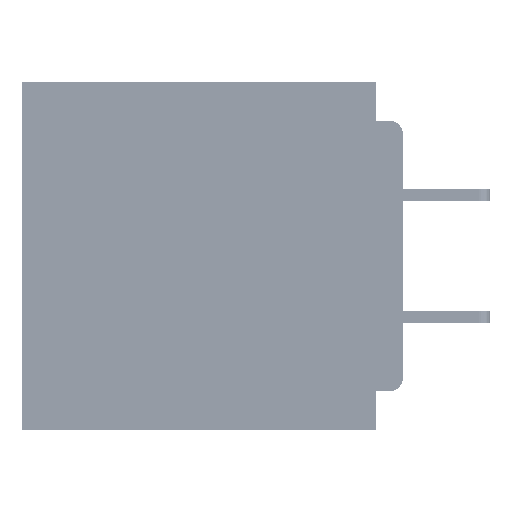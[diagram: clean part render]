
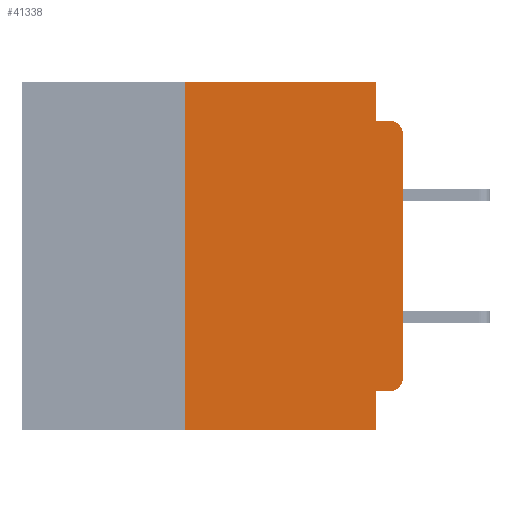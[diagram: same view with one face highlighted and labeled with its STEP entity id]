
A CAD part, left-side view. The second image highlights one B-rep face of the part: STEP entity #41338.
In plain terms, the highlighted planar face has unit normal (-1, 0, 0).
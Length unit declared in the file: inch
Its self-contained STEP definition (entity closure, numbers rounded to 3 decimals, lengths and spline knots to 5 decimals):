
#2596 = LINE ( 'NONE', #50069, #58833 ) ;
#3687 = DIRECTION ( 'NONE',  ( 0., 0., -1. ) ) ;
#3823 = CIRCLE ( 'NONE', #4908, 0.015 ) ;
#4255 = VERTEX_POINT ( 'NONE', #46922 ) ;
#4647 = DIRECTION ( 'NONE',  ( 0., 0., 1. ) ) ;
#4908 = AXIS2_PLACEMENT_3D ( 'NONE', #70573, #38184, #5376 ) ;
#5376 = DIRECTION ( 'NONE',  ( 0., 0., -1. ) ) ;
#5765 = VECTOR ( 'NONE', #49019, 39.37008 ) ;
#6104 = VECTOR ( 'NONE', #42588, 39.37008 ) ;
#8023 = VERTEX_POINT ( 'NONE', #57097 ) ;
#11063 = ORIENTED_EDGE ( 'NONE', *, *, #49867, .T. ) ;
#13191 = ORIENTED_EDGE ( 'NONE', *, *, #67345, .F. ) ;
#15034 = CIRCLE ( 'NONE', #28139, 0.015 ) ;
#16459 = CARTESIAN_POINT ( 'NONE',  ( 0., 0.25, -0.4 ) ) ;
#16585 = EDGE_LOOP ( 'NONE', ( #11063, #57683, #36805, #46174, #51348, #13191, #30051, #34677, #66850, #38359 ) ) ;
#17734 = DIRECTION ( 'NONE',  ( 1., 0., 0. ) ) ;
#17931 = VECTOR ( 'NONE', #3687, 39.37008 ) ;
#18773 = CARTESIAN_POINT ( 'NONE',  ( 0., 0.25, -0.4 ) ) ;
#18894 = CARTESIAN_POINT ( 'NONE',  ( 0., 0.015, -0.34 ) ) ;
#18931 = LINE ( 'NONE', #30530, #46147 ) ;
#20295 = CARTESIAN_POINT ( 'NONE',  ( 0., 0.031, -0.4 ) ) ;
#20372 = LINE ( 'NONE', #27208, #5765 ) ;
#21933 = EDGE_CURVE ( 'NONE', #69608, #4255, #18931, .T. ) ;
#21952 = DIRECTION ( 'NONE',  ( 0., 0., 1. ) ) ;
#22398 = CARTESIAN_POINT ( 'NONE',  ( 0., 0.015, -0.045 ) ) ;
#23868 = VERTEX_POINT ( 'NONE', #22398 ) ;
#24397 = DIRECTION ( 'NONE',  ( 0., 0., -1. ) ) ;
#26421 = VERTEX_POINT ( 'NONE', #55710 ) ;
#26506 = CARTESIAN_POINT ( 'NONE',  ( 0., 0., 0. ) ) ;
#27208 = CARTESIAN_POINT ( 'NONE',  ( 0., 0.437, 0. ) ) ;
#27785 = LINE ( 'NONE', #61998, #38834 ) ;
#28139 = AXIS2_PLACEMENT_3D ( 'NONE', #18894, #56867, #24397 ) ;
#29592 = DIRECTION ( 'NONE',  ( 0., -1., 0. ) ) ;
#30051 = ORIENTED_EDGE ( 'NONE', *, *, #55115, .T. ) ;
#30530 = CARTESIAN_POINT ( 'NONE',  ( 0., 0., -0.355 ) ) ;
#30742 = LINE ( 'NONE', #20295, #17931 ) ;
#30955 = VERTEX_POINT ( 'NONE', #55460 ) ;
#32344 = CARTESIAN_POINT ( 'NONE',  ( 0., 0.031, -0.4 ) ) ;
#34677 = ORIENTED_EDGE ( 'NONE', *, *, #67169, .F. ) ;
#35295 = LINE ( 'NONE', #64104, #6104 ) ;
#36805 = ORIENTED_EDGE ( 'NONE', *, *, #61801, .F. ) ;
#38006 = VERTEX_POINT ( 'NONE', #18773 ) ;
#38184 = DIRECTION ( 'NONE',  ( -1., 0., 0. ) ) ;
#38359 = ORIENTED_EDGE ( 'NONE', *, *, #49591, .T. ) ;
#38834 = VECTOR ( 'NONE', #29592, 39.37008 ) ;
#39362 = VERTEX_POINT ( 'NONE', #47837 ) ;
#39425 = CARTESIAN_POINT ( 'NONE',  ( 0., 0.437, 0. ) ) ;
#41338 = ADVANCED_FACE ( 'NONE', ( #51586 ), #50280, .F. ) ;
#41408 = VECTOR ( 'NONE', #4647, 39.37008 ) ;
#42130 = CARTESIAN_POINT ( 'NONE',  ( 0., 0.031, -0.045 ) ) ;
#42588 = DIRECTION ( 'NONE',  ( 0., 0., -1. ) ) ;
#45502 = CARTESIAN_POINT ( 'NONE',  ( 0., 0.015, -0.355 ) ) ;
#46147 = VECTOR ( 'NONE', #47123, 39.37008 ) ;
#46174 = ORIENTED_EDGE ( 'NONE', *, *, #52191, .F. ) ;
#46922 = CARTESIAN_POINT ( 'NONE',  ( 0., 0.031, -0.355 ) ) ;
#47123 = DIRECTION ( 'NONE',  ( 0., 1., 0. ) ) ;
#47837 = CARTESIAN_POINT ( 'NONE',  ( 0., 0.031, 0. ) ) ;
#49019 = DIRECTION ( 'NONE',  ( 0., -1., 0. ) ) ;
#49591 = EDGE_CURVE ( 'NONE', #69608, #8023, #15034, .T. ) ;
#49867 = EDGE_CURVE ( 'NONE', #8023, #26421, #68522, .T. ) ;
#50069 = CARTESIAN_POINT ( 'NONE',  ( 0., 0., -0.045 ) ) ;
#50280 = PLANE ( 'NONE',  #51409 ) ;
#51065 = LINE ( 'NONE', #16459, #62050 ) ;
#51348 = ORIENTED_EDGE ( 'NONE', *, *, #58600, .F. ) ;
#51409 = AXIS2_PLACEMENT_3D ( 'NONE', #39425, #17734, #55713 ) ;
#51586 = FACE_OUTER_BOUND ( 'NONE', #16585, .T. ) ;
#52191 = EDGE_CURVE ( 'NONE', #39362, #55306, #35295, .T. ) ;
#55115 = EDGE_CURVE ( 'NONE', #38006, #65452, #27785, .T. ) ;
#55306 = VERTEX_POINT ( 'NONE', #42130 ) ;
#55460 = CARTESIAN_POINT ( 'NONE',  ( 0., 0.25, 0. ) ) ;
#55503 = DIRECTION ( 'NONE',  ( 0., -1., 0. ) ) ;
#55710 = CARTESIAN_POINT ( 'NONE',  ( 0., 0., -0.06 ) ) ;
#55713 = DIRECTION ( 'NONE',  ( 0., 0., -1. ) ) ;
#56867 = DIRECTION ( 'NONE',  ( -1., 0., 0. ) ) ;
#57097 = CARTESIAN_POINT ( 'NONE',  ( 0., 0., -0.34 ) ) ;
#57683 = ORIENTED_EDGE ( 'NONE', *, *, #69221, .T. ) ;
#58600 = EDGE_CURVE ( 'NONE', #30955, #39362, #20372, .T. ) ;
#58833 = VECTOR ( 'NONE', #55503, 39.37008 ) ;
#61801 = EDGE_CURVE ( 'NONE', #55306, #23868, #2596, .T. ) ;
#61998 = CARTESIAN_POINT ( 'NONE',  ( 0., 0.437, -0.4 ) ) ;
#62050 = VECTOR ( 'NONE', #21952, 39.37008 ) ;
#64104 = CARTESIAN_POINT ( 'NONE',  ( 0., 0.031, 0. ) ) ;
#65452 = VERTEX_POINT ( 'NONE', #32344 ) ;
#66850 = ORIENTED_EDGE ( 'NONE', *, *, #21933, .F. ) ;
#67169 = EDGE_CURVE ( 'NONE', #4255, #65452, #30742, .T. ) ;
#67345 = EDGE_CURVE ( 'NONE', #38006, #30955, #51065, .T. ) ;
#68522 = LINE ( 'NONE', #26506, #41408 ) ;
#69221 = EDGE_CURVE ( 'NONE', #26421, #23868, #3823, .T. ) ;
#69608 = VERTEX_POINT ( 'NONE', #45502 ) ;
#70573 = CARTESIAN_POINT ( 'NONE',  ( 0., 0.015, -0.06 ) ) ;
